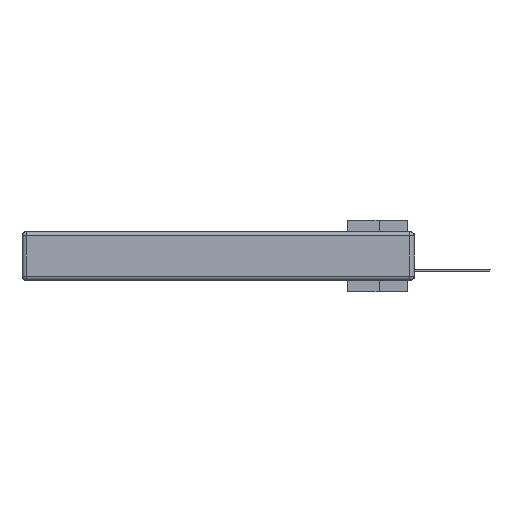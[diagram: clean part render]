
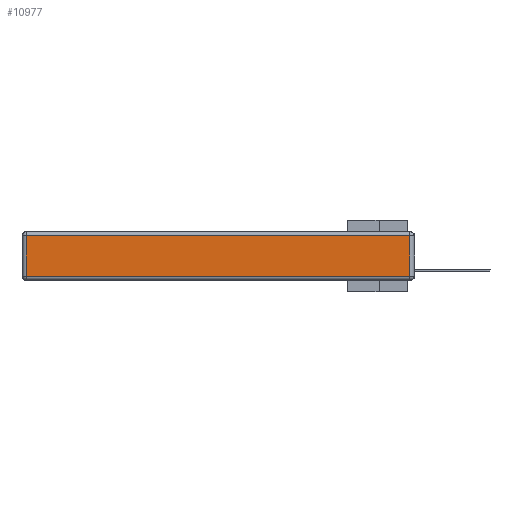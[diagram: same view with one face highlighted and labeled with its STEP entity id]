
A CAD part, left-side view. The second image highlights one B-rep face of the part: STEP entity #10977.
In plain terms, the highlighted planar face has unit normal (-1, 0, 0).
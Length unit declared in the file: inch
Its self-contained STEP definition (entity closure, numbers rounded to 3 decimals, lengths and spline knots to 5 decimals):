
#1539 = PLANE ( 'NONE',  #9596 ) ;
#2163 = DIRECTION ( 'NONE',  ( 0., 0., 1. ) ) ;
#3311 = CARTESIAN_POINT ( 'NONE',  ( 0., 2.72, -0.313 ) ) ;
#5148 = ORIENTED_EDGE ( 'NONE', *, *, #17542, .T. ) ;
#5253 = DIRECTION ( 'NONE',  ( 0., -1., 0. ) ) ;
#5335 = VECTOR ( 'NONE', #23755, 39.37008 ) ;
#5637 = EDGE_CURVE ( 'NONE', #19534, #29726, #7859, .T. ) ;
#6990 = DIRECTION ( 'NONE',  ( 0., 1., 0. ) ) ;
#7859 = LINE ( 'NONE', #25403, #29673 ) ;
#9596 = AXIS2_PLACEMENT_3D ( 'NONE', #14529, #24425, #2163 ) ;
#10164 = LINE ( 'NONE', #27223, #23957 ) ;
#10977 = ADVANCED_FACE ( 'NONE', ( #16955 ), #1539, .T. ) ;
#11237 = EDGE_LOOP ( 'NONE', ( #15418, #5148, #31102, #15147 ) ) ;
#11335 = VECTOR ( 'NONE', #6990, 39.37008 ) ;
#12781 = EDGE_CURVE ( 'NONE', #19522, #19534, #31081, .T. ) ;
#14529 = CARTESIAN_POINT ( 'NONE',  ( 0., 0., -0.343 ) ) ;
#15147 = ORIENTED_EDGE ( 'NONE', *, *, #12781, .T. ) ;
#15418 = ORIENTED_EDGE ( 'NONE', *, *, #5637, .T. ) ;
#15693 = CARTESIAN_POINT ( 'NONE',  ( 0., 0.03, -0.03 ) ) ;
#16734 = VERTEX_POINT ( 'NONE', #15693 ) ;
#16955 = FACE_OUTER_BOUND ( 'NONE', #11237, .T. ) ;
#17542 = EDGE_CURVE ( 'NONE', #29726, #16734, #10164, .T. ) ;
#19522 = VERTEX_POINT ( 'NONE', #28163 ) ;
#19534 = VERTEX_POINT ( 'NONE', #3311 ) ;
#19599 = DIRECTION ( 'NONE',  ( 0., 0., 1. ) ) ;
#21424 = EDGE_CURVE ( 'NONE', #16734, #19522, #31696, .T. ) ;
#21925 = CARTESIAN_POINT ( 'NONE',  ( 0., 2.75, -0.03 ) ) ;
#23755 = DIRECTION ( 'NONE',  ( 0., 0., -1. ) ) ;
#23957 = VECTOR ( 'NONE', #19599, 39.37008 ) ;
#24425 = DIRECTION ( 'NONE',  ( -1., 0., 0. ) ) ;
#25403 = CARTESIAN_POINT ( 'NONE',  ( 0., 0., -0.313 ) ) ;
#27223 = CARTESIAN_POINT ( 'NONE',  ( 0., 0.03, -0.343 ) ) ;
#28163 = CARTESIAN_POINT ( 'NONE',  ( 0., 2.72, -0.03 ) ) ;
#28629 = CARTESIAN_POINT ( 'NONE',  ( 0., 2.72, -0.343 ) ) ;
#29673 = VECTOR ( 'NONE', #5253, 39.37008 ) ;
#29726 = VERTEX_POINT ( 'NONE', #31618 ) ;
#31081 = LINE ( 'NONE', #28629, #5335 ) ;
#31102 = ORIENTED_EDGE ( 'NONE', *, *, #21424, .T. ) ;
#31618 = CARTESIAN_POINT ( 'NONE',  ( 0., 0.03, -0.313 ) ) ;
#31696 = LINE ( 'NONE', #21925, #11335 ) ;
